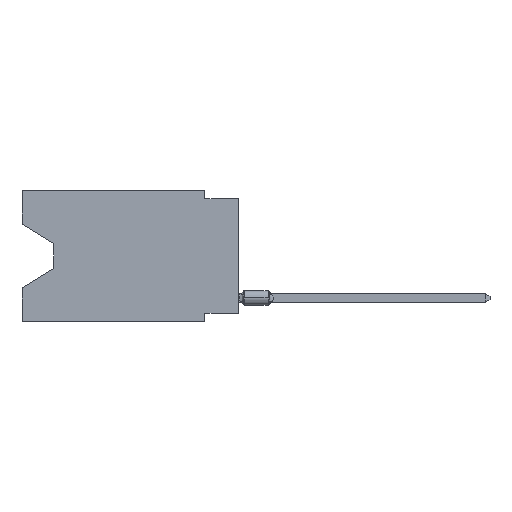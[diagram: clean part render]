
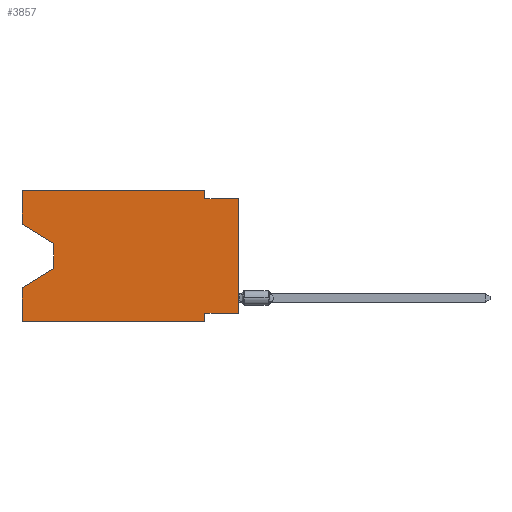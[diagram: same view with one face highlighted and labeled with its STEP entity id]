
A CAD part, left-side view. The second image highlights one B-rep face of the part: STEP entity #3857.
In plain terms, the highlighted planar face has unit normal (-1, 0, 0).
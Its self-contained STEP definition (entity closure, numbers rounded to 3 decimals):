
#152 = AXIS2_PLACEMENT_3D ( 'NONE', #8911, #10136, #10012 ) ;
#240 = EDGE_CURVE ( 'NONE', #7774, #3995, #11179, .T. ) ;
#366 = CARTESIAN_POINT ( 'NONE',  ( 0., 0., -9.271 ) ) ;
#421 = VERTEX_POINT ( 'NONE', #1765 ) ;
#556 = VECTOR ( 'NONE', #5757, 1000. ) ;
#597 = CARTESIAN_POINT ( 'NONE',  ( 0., 16.383, -7.36 ) ) ;
#785 = DIRECTION ( 'NONE',  ( 0., 0., 1. ) ) ;
#1048 = CARTESIAN_POINT ( 'NONE',  ( 0., 0., 0. ) ) ;
#1214 = VERTEX_POINT ( 'NONE', #4057 ) ;
#1327 = ORIENTED_EDGE ( 'NONE', *, *, #3862, .T. ) ;
#1517 = VERTEX_POINT ( 'NONE', #597 ) ;
#1600 = ORIENTED_EDGE ( 'NONE', *, *, #240, .F. ) ;
#1765 = CARTESIAN_POINT ( 'NONE',  ( 0., 16.383, -9.906 ) ) ;
#1790 = EDGE_LOOP ( 'NONE', ( #8083, #1327, #9804, #3422, #5655, #11294, #4993, #7262, #12152, #3269, #1600, #6254 ) ) ;
#1828 = VECTOR ( 'NONE', #5225, 1000. ) ;
#2255 = DIRECTION ( 'NONE',  ( 0., 1., 0. ) ) ;
#2576 = VECTOR ( 'NONE', #785, 1000. ) ;
#2664 = VERTEX_POINT ( 'NONE', #7360 ) ;
#2867 = VERTEX_POINT ( 'NONE', #6967 ) ;
#2941 = LINE ( 'NONE', #8767, #4369 ) ;
#3011 = PLANE ( 'NONE',  #152 ) ;
#3111 = VECTOR ( 'NONE', #2255, 1000. ) ;
#3267 = VECTOR ( 'NONE', #3505, 1000. ) ;
#3269 = ORIENTED_EDGE ( 'NONE', *, *, #8371, .F. ) ;
#3422 = ORIENTED_EDGE ( 'NONE', *, *, #4997, .F. ) ;
#3505 = DIRECTION ( 'NONE',  ( 0., 0., -1. ) ) ;
#3810 = EDGE_CURVE ( 'NONE', #3993, #2867, #4879, .T. ) ;
#3857 = ADVANCED_FACE ( 'NONE', ( #11890 ), #3011, .F. ) ;
#3862 = EDGE_CURVE ( 'NONE', #9590, #10789, #8054, .T. ) ;
#3914 = DIRECTION ( 'NONE',  ( 0., -1., 0. ) ) ;
#3993 = VERTEX_POINT ( 'NONE', #12214 ) ;
#3995 = VERTEX_POINT ( 'NONE', #12338 ) ;
#4057 = CARTESIAN_POINT ( 'NONE',  ( 0., 2.54, -9.271 ) ) ;
#4073 = LINE ( 'NONE', #9067, #3267 ) ;
#4220 = CARTESIAN_POINT ( 'NONE',  ( 0., 16.383, -2.546 ) ) ;
#4369 = VECTOR ( 'NONE', #6699, 1000. ) ;
#4554 = EDGE_CURVE ( 'NONE', #421, #2664, #10697, .T. ) ;
#4675 = EDGE_CURVE ( 'NONE', #1214, #2664, #4073, .T. ) ;
#4879 = LINE ( 'NONE', #12796, #9246 ) ;
#4993 = ORIENTED_EDGE ( 'NONE', *, *, #7442, .F. ) ;
#4997 = EDGE_CURVE ( 'NONE', #421, #1517, #5617, .T. ) ;
#5225 = DIRECTION ( 'NONE',  ( 0., -0.855, -0.519 ) ) ;
#5265 = CARTESIAN_POINT ( 'NONE',  ( 0., 2.54, 0. ) ) ;
#5333 = DIRECTION ( 'NONE',  ( 0., -1., 0. ) ) ;
#5587 = VECTOR ( 'NONE', #5333, 1000. ) ;
#5617 = LINE ( 'NONE', #5676, #11760 ) ;
#5646 = EDGE_CURVE ( 'NONE', #12242, #9590, #9123, .T. ) ;
#5655 = ORIENTED_EDGE ( 'NONE', *, *, #4554, .T. ) ;
#5676 = CARTESIAN_POINT ( 'NONE',  ( 0., 16.383, 0. ) ) ;
#5709 = LINE ( 'NONE', #6703, #2576 ) ;
#5757 = DIRECTION ( 'NONE',  ( 0., -1., 0. ) ) ;
#6147 = VECTOR ( 'NONE', #9159, 1000. ) ;
#6254 = ORIENTED_EDGE ( 'NONE', *, *, #12119, .F. ) ;
#6301 = DIRECTION ( 'NONE',  ( 0., 0., -1. ) ) ;
#6699 = DIRECTION ( 'NONE',  ( 0., 0.855, -0.519 ) ) ;
#6703 = CARTESIAN_POINT ( 'NONE',  ( 0., 16.383, 0. ) ) ;
#6905 = CARTESIAN_POINT ( 'NONE',  ( 0., 13.97, -4.013 ) ) ;
#6924 = CARTESIAN_POINT ( 'NONE',  ( 0., 16.383, 0. ) ) ;
#6967 = CARTESIAN_POINT ( 'NONE',  ( 0., 0., -0.635 ) ) ;
#7262 = ORIENTED_EDGE ( 'NONE', *, *, #9378, .T. ) ;
#7360 = CARTESIAN_POINT ( 'NONE',  ( 0., 2.54, -9.906 ) ) ;
#7434 = DIRECTION ( 'NONE',  ( 0., 0., 1. ) ) ;
#7442 = EDGE_CURVE ( 'NONE', #10250, #1214, #8350, .T. ) ;
#7774 = VERTEX_POINT ( 'NONE', #6924 ) ;
#7791 = LINE ( 'NONE', #1048, #11601 ) ;
#8054 = LINE ( 'NONE', #6905, #6147 ) ;
#8083 = ORIENTED_EDGE ( 'NONE', *, *, #5646, .T. ) ;
#8324 = LINE ( 'NONE', #5265, #10576 ) ;
#8350 = LINE ( 'NONE', #366, #3111 ) ;
#8371 = EDGE_CURVE ( 'NONE', #3995, #3993, #8324, .T. ) ;
#8560 = CARTESIAN_POINT ( 'NONE',  ( 0., 13.97, -4.013 ) ) ;
#8621 = EDGE_CURVE ( 'NONE', #10789, #1517, #2941, .T. ) ;
#8767 = CARTESIAN_POINT ( 'NONE',  ( 0., 13.97, -5.893 ) ) ;
#8911 = CARTESIAN_POINT ( 'NONE',  ( 0., 16.383, 0. ) ) ;
#8962 = DIRECTION ( 'NONE',  ( 0., 0., 1. ) ) ;
#9067 = CARTESIAN_POINT ( 'NONE',  ( 0., 2.54, -9.906 ) ) ;
#9123 = LINE ( 'NONE', #11915, #1828 ) ;
#9159 = DIRECTION ( 'NONE',  ( 0., 0., -1. ) ) ;
#9246 = VECTOR ( 'NONE', #3914, 1000. ) ;
#9378 = EDGE_CURVE ( 'NONE', #10250, #2867, #7791, .T. ) ;
#9590 = VERTEX_POINT ( 'NONE', #8560 ) ;
#9804 = ORIENTED_EDGE ( 'NONE', *, *, #8621, .T. ) ;
#10012 = DIRECTION ( 'NONE',  ( 0., 0., -1. ) ) ;
#10136 = DIRECTION ( 'NONE',  ( 1., 0., 0. ) ) ;
#10222 = CARTESIAN_POINT ( 'NONE',  ( 0., 0., -9.271 ) ) ;
#10250 = VERTEX_POINT ( 'NONE', #10222 ) ;
#10272 = CARTESIAN_POINT ( 'NONE',  ( 0., 16.383, 0. ) ) ;
#10576 = VECTOR ( 'NONE', #6301, 1000. ) ;
#10697 = LINE ( 'NONE', #11475, #556 ) ;
#10789 = VERTEX_POINT ( 'NONE', #11672 ) ;
#11179 = LINE ( 'NONE', #10272, #5587 ) ;
#11294 = ORIENTED_EDGE ( 'NONE', *, *, #4675, .F. ) ;
#11475 = CARTESIAN_POINT ( 'NONE',  ( 0., 16.383, -9.906 ) ) ;
#11601 = VECTOR ( 'NONE', #8962, 1000. ) ;
#11672 = CARTESIAN_POINT ( 'NONE',  ( 0., 13.97, -5.893 ) ) ;
#11760 = VECTOR ( 'NONE', #7434, 1000. ) ;
#11890 = FACE_OUTER_BOUND ( 'NONE', #1790, .T. ) ;
#11915 = CARTESIAN_POINT ( 'NONE',  ( 0., 16.383, -2.546 ) ) ;
#12119 = EDGE_CURVE ( 'NONE', #12242, #7774, #5709, .T. ) ;
#12152 = ORIENTED_EDGE ( 'NONE', *, *, #3810, .F. ) ;
#12214 = CARTESIAN_POINT ( 'NONE',  ( 0., 2.54, -0.635 ) ) ;
#12242 = VERTEX_POINT ( 'NONE', #4220 ) ;
#12338 = CARTESIAN_POINT ( 'NONE',  ( 0., 2.54, 0. ) ) ;
#12796 = CARTESIAN_POINT ( 'NONE',  ( 0., 0., -0.635 ) ) ;
